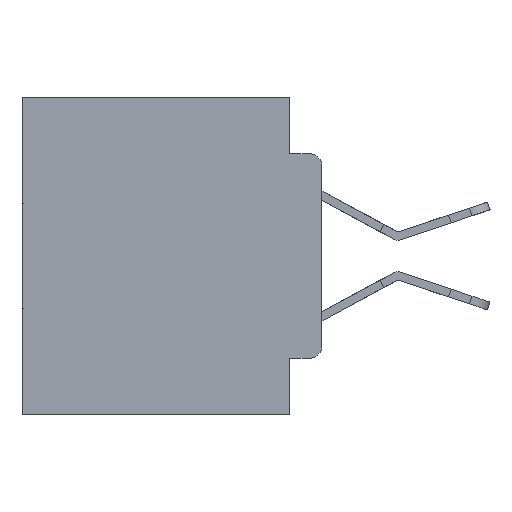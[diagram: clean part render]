
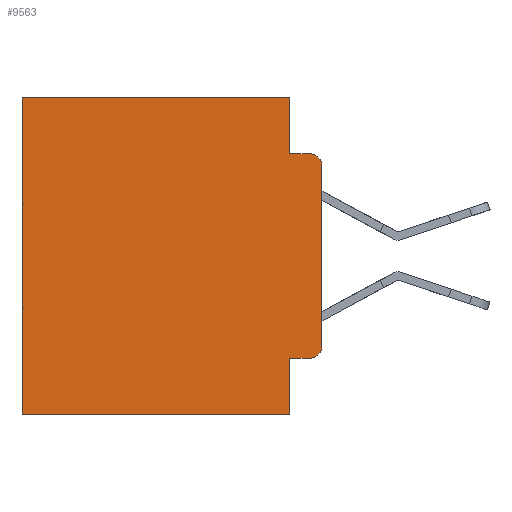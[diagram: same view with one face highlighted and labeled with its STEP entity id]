
A CAD part, left-side view. The second image highlights one B-rep face of the part: STEP entity #9563.
In plain terms, the highlighted planar face has unit normal (-1, 0, 0).
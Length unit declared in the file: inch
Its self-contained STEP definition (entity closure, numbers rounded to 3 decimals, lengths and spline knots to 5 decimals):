
#643 = ORIENTED_EDGE ( 'NONE', *, *, #12490, .T. ) ;
#1482 = DIRECTION ( 'NONE',  ( 0., -1., 0. ) ) ;
#2646 = CARTESIAN_POINT ( 'NONE',  ( 0.298, 0.02, -0.3915 ) ) ;
#2912 = VECTOR ( 'NONE', #22173, 39.37008 ) ;
#3211 = VECTOR ( 'NONE', #25567, 39.37008 ) ;
#3572 = CARTESIAN_POINT ( 'NONE',  ( 0.298, 0.02, -0.1085 ) ) ;
#4036 = VERTEX_POINT ( 'NONE', #18286 ) ;
#4073 = CARTESIAN_POINT ( 'NONE',  ( 0.298, 0.051, -0.4115 ) ) ;
#4437 = AXIS2_PLACEMENT_3D ( 'NONE', #3572, #20700, #10914 ) ;
#4645 = EDGE_CURVE ( 'NONE', #15742, #20543, #29322, .T. ) ;
#5112 = DIRECTION ( 'NONE',  ( 0., 0., -1. ) ) ;
#5163 = VERTEX_POINT ( 'NONE', #15242 ) ;
#5250 = LINE ( 'NONE', #30048, #28268 ) ;
#5437 = FACE_OUTER_BOUND ( 'NONE', #24387, .T. ) ;
#5514 = ORIENTED_EDGE ( 'NONE', *, *, #15984, .T. ) ;
#5547 = DIRECTION ( 'NONE',  ( 0., -1., 0. ) ) ;
#5875 = CARTESIAN_POINT ( 'NONE',  ( 0.298, 0.051, -0.4115 ) ) ;
#6652 = ORIENTED_EDGE ( 'NONE', *, *, #32133, .T. ) ;
#7728 = PLANE ( 'NONE',  #30564 ) ;
#7876 = DIRECTION ( 'NONE',  ( -1., 0., 0. ) ) ;
#9081 = CARTESIAN_POINT ( 'NONE',  ( 0.298, 0.02, -0.4115 ) ) ;
#9563 = ADVANCED_FACE ( 'NONE', ( #5437 ), #7728, .F. ) ;
#10205 = CARTESIAN_POINT ( 'NONE',  ( 0.298, 0., 0. ) ) ;
#10914 = DIRECTION ( 'NONE',  ( 0., 0., -1. ) ) ;
#11436 = CARTESIAN_POINT ( 'NONE',  ( 0.298, 0.051, -0.0885 ) ) ;
#11508 = EDGE_CURVE ( 'NONE', #24944, #26013, #15517, .T. ) ;
#12027 = DIRECTION ( 'NONE',  ( 0., 0., -1. ) ) ;
#12490 = EDGE_CURVE ( 'NONE', #24944, #19326, #29954, .T. ) ;
#12903 = DIRECTION ( 'NONE',  ( 0., 0., -1. ) ) ;
#13457 = CARTESIAN_POINT ( 'NONE',  ( 0.298, 0.051, -0.0885 ) ) ;
#13589 = ORIENTED_EDGE ( 'NONE', *, *, #30103, .T. ) ;
#14492 = LINE ( 'NONE', #24430, #2912 ) ;
#14530 = VERTEX_POINT ( 'NONE', #9081 ) ;
#14647 = ORIENTED_EDGE ( 'NONE', *, *, #22085, .F. ) ;
#15242 = CARTESIAN_POINT ( 'NONE',  ( 0.298, 0.473, -0.5 ) ) ;
#15244 = EDGE_CURVE ( 'NONE', #18543, #19326, #23994, .T. ) ;
#15517 = LINE ( 'NONE', #25428, #19660 ) ;
#15742 = VERTEX_POINT ( 'NONE', #4073 ) ;
#15984 = EDGE_CURVE ( 'NONE', #4036, #20942, #22285, .T. ) ;
#16564 = VECTOR ( 'NONE', #1482, 39.37008 ) ;
#16702 = ORIENTED_EDGE ( 'NONE', *, *, #28861, .F. ) ;
#17866 = DIRECTION ( 'NONE',  ( 0., 1., 0. ) ) ;
#18091 = CARTESIAN_POINT ( 'NONE',  ( 0.298, 0., -0.1085 ) ) ;
#18286 = CARTESIAN_POINT ( 'NONE',  ( 0.298, 0.051, 0. ) ) ;
#18543 = VERTEX_POINT ( 'NONE', #13457 ) ;
#18608 = VECTOR ( 'NONE', #17866, 39.37008 ) ;
#18802 = ORIENTED_EDGE ( 'NONE', *, *, #15244, .F. ) ;
#19326 = VERTEX_POINT ( 'NONE', #19740 ) ;
#19489 = EDGE_CURVE ( 'NONE', #15742, #14530, #30502, .T. ) ;
#19660 = VECTOR ( 'NONE', #12903, 39.37008 ) ;
#19740 = CARTESIAN_POINT ( 'NONE',  ( 0.298, 0.02, -0.0885 ) ) ;
#20543 = VERTEX_POINT ( 'NONE', #30692 ) ;
#20700 = DIRECTION ( 'NONE',  ( -1., 0., 0. ) ) ;
#20942 = VERTEX_POINT ( 'NONE', #30980 ) ;
#22085 = EDGE_CURVE ( 'NONE', #20543, #5163, #25242, .T. ) ;
#22173 = DIRECTION ( 'NONE',  ( 0., 0., -1. ) ) ;
#22285 = LINE ( 'NONE', #10205, #18608 ) ;
#22741 = DIRECTION ( 'NONE',  ( 0., 0., -1. ) ) ;
#23068 = ORIENTED_EDGE ( 'NONE', *, *, #4645, .F. ) ;
#23937 = ORIENTED_EDGE ( 'NONE', *, *, #11508, .F. ) ;
#23988 = VECTOR ( 'NONE', #12027, 39.37008 ) ;
#23994 = LINE ( 'NONE', #11436, #16564 ) ;
#24365 = ORIENTED_EDGE ( 'NONE', *, *, #19489, .T. ) ;
#24387 = EDGE_LOOP ( 'NONE', ( #23937, #643, #18802, #16702, #5514, #6652, #14647, #23068, #24365, #13589 ) ) ;
#24430 = CARTESIAN_POINT ( 'NONE',  ( 0.298, 0.473, 0. ) ) ;
#24944 = VERTEX_POINT ( 'NONE', #18091 ) ;
#25242 = LINE ( 'NONE', #30492, #3211 ) ;
#25428 = CARTESIAN_POINT ( 'NONE',  ( 0.298, 0., 0. ) ) ;
#25567 = DIRECTION ( 'NONE',  ( 0., 1., 0. ) ) ;
#26013 = VERTEX_POINT ( 'NONE', #28924 ) ;
#27451 = DIRECTION ( 'NONE',  ( 1., 0., 0. ) ) ;
#27915 = DIRECTION ( 'NONE',  ( 0., 0., -1. ) ) ;
#28268 = VECTOR ( 'NONE', #27915, 39.37008 ) ;
#28861 = EDGE_CURVE ( 'NONE', #4036, #18543, #5250, .T. ) ;
#28924 = CARTESIAN_POINT ( 'NONE',  ( 0.298, 0., -0.3915 ) ) ;
#29015 = CARTESIAN_POINT ( 'NONE',  ( 0.298, 0.051, 0. ) ) ;
#29322 = LINE ( 'NONE', #29015, #23988 ) ;
#29393 = AXIS2_PLACEMENT_3D ( 'NONE', #2646, #7876, #22741 ) ;
#29912 = CARTESIAN_POINT ( 'NONE',  ( 0.298, 0., 0. ) ) ;
#29954 = CIRCLE ( 'NONE', #4437, 0.02 ) ;
#30048 = CARTESIAN_POINT ( 'NONE',  ( 0.298, 0.051, 0. ) ) ;
#30103 = EDGE_CURVE ( 'NONE', #14530, #26013, #31488, .T. ) ;
#30492 = CARTESIAN_POINT ( 'NONE',  ( 0.298, 0., -0.5 ) ) ;
#30502 = LINE ( 'NONE', #5875, #31276 ) ;
#30564 = AXIS2_PLACEMENT_3D ( 'NONE', #29912, #27451, #5112 ) ;
#30692 = CARTESIAN_POINT ( 'NONE',  ( 0.298, 0.051, -0.5 ) ) ;
#30980 = CARTESIAN_POINT ( 'NONE',  ( 0.298, 0.473, 0. ) ) ;
#31276 = VECTOR ( 'NONE', #5547, 39.37008 ) ;
#31488 = CIRCLE ( 'NONE', #29393, 0.02 ) ;
#32133 = EDGE_CURVE ( 'NONE', #20942, #5163, #14492, .T. ) ;
